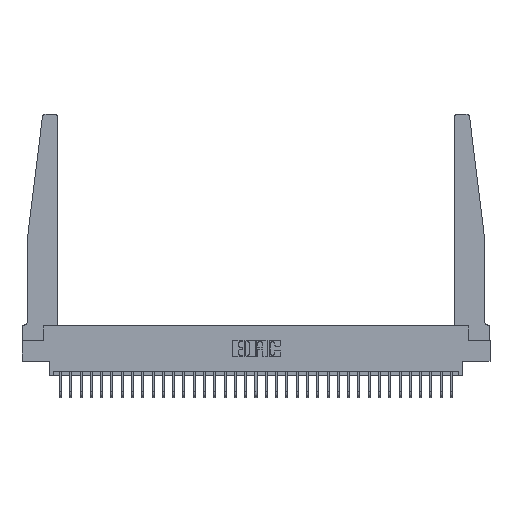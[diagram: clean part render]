
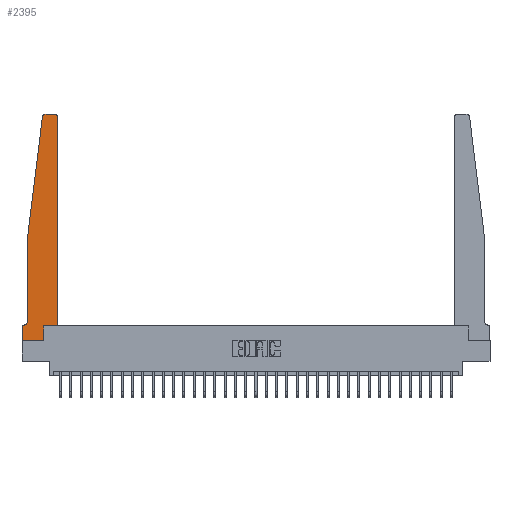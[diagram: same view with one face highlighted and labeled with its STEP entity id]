
A CAD part, top view. The second image highlights one B-rep face of the part: STEP entity #2395.
In plain terms, the highlighted planar face has unit normal (0, 0, 1).
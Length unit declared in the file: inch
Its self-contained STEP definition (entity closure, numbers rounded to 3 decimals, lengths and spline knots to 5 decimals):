
#1 = EDGE_CURVE ( 'NONE', #13689, #23639, #2510, .T. ) ;
#8 = DIRECTION ( 'NONE',  ( 0., 0., 1. ) ) ;
#1365 = ORIENTED_EDGE ( 'NONE', *, *, #23970, .T. ) ;
#1791 = EDGE_LOOP ( 'NONE', ( #9352, #6189, #14018, #2308, #9641, #16532, #23298, #17718, #9999, #11771, #1365, #20851 ) ) ;
#2158 = VERTEX_POINT ( 'NONE', #26513 ) ;
#2192 = DIRECTION ( 'NONE',  ( 0., 1., 0. ) ) ;
#2308 = ORIENTED_EDGE ( 'NONE', *, *, #10575, .T. ) ;
#2395 = ADVANCED_FACE ( 'NONE', ( #23514 ), #27385, .T. ) ;
#2459 = DIRECTION ( 'NONE',  ( -1., 0., 0. ) ) ;
#2510 = LINE ( 'NONE', #25712, #26073 ) ;
#2890 = AXIS2_PLACEMENT_3D ( 'NONE', #27079, #13449, #29350 ) ;
#3058 = VECTOR ( 'NONE', #11394, 39.37008 ) ;
#3444 = CARTESIAN_POINT ( 'NONE',  ( 0.015, 0.2375, 0.37 ) ) ;
#4073 = CARTESIAN_POINT ( 'NONE',  ( 0., 0., 0.37 ) ) ;
#4116 = EDGE_CURVE ( 'NONE', #18996, #13689, #15568, .T. ) ;
#4130 = AXIS2_PLACEMENT_3D ( 'NONE', #3444, #19445, #5785 ) ;
#5109 = VECTOR ( 'NONE', #2192, 39.37008 ) ;
#5785 = DIRECTION ( 'NONE',  ( -1., 0., 0. ) ) ;
#6189 = ORIENTED_EDGE ( 'NONE', *, *, #13111, .T. ) ;
#6371 = LINE ( 'NONE', #24095, #13177 ) ;
#6589 = EDGE_CURVE ( 'NONE', #14719, #13259, #29005, .T. ) ;
#7492 = CARTESIAN_POINT ( 'NONE',  ( 0.065, 1.25, 0.37 ) ) ;
#8091 = CARTESIAN_POINT ( 'NONE',  ( 0.395, 2.72, 0.37 ) ) ;
#8122 = DIRECTION ( 'NONE',  ( 0., -1., 0. ) ) ;
#8791 = VECTOR ( 'NONE', #26697, 39.37008 ) ;
#9352 = ORIENTED_EDGE ( 'NONE', *, *, #25266, .T. ) ;
#9641 = ORIENTED_EDGE ( 'NONE', *, *, #17659, .T. ) ;
#9794 = EDGE_CURVE ( 'NONE', #13259, #18996, #6371, .T. ) ;
#9999 = ORIENTED_EDGE ( 'NONE', *, *, #1, .T. ) ;
#10237 = DIRECTION ( 'NONE',  ( 1., 0., 0. ) ) ;
#10416 = DIRECTION ( 'NONE',  ( 1., 0., 0. ) ) ;
#10575 = EDGE_CURVE ( 'NONE', #20469, #19126, #15935, .T. ) ;
#11394 = DIRECTION ( 'NONE',  ( 0., -1., 0. ) ) ;
#11771 = ORIENTED_EDGE ( 'NONE', *, *, #29094, .T. ) ;
#11962 = EDGE_CURVE ( 'NONE', #21067, #12839, #21216, .T. ) ;
#12839 = VERTEX_POINT ( 'NONE', #27115 ) ;
#13071 = CARTESIAN_POINT ( 'NONE',  ( 0., 0., 0.37 ) ) ;
#13111 = EDGE_CURVE ( 'NONE', #2158, #23905, #21515, .T. ) ;
#13177 = VECTOR ( 'NONE', #8122, 39.37008 ) ;
#13259 = VERTEX_POINT ( 'NONE', #13929 ) ;
#13449 = DIRECTION ( 'NONE',  ( 0., 0., 1. ) ) ;
#13612 = CARTESIAN_POINT ( 'NONE',  ( 0.425, 0.18, 0.37 ) ) ;
#13689 = VERTEX_POINT ( 'NONE', #17655 ) ;
#13705 = CARTESIAN_POINT ( 'NONE',  ( 0.065, 0.2375, 0.37 ) ) ;
#13807 = VERTEX_POINT ( 'NONE', #13612 ) ;
#13882 = CARTESIAN_POINT ( 'NONE',  ( 0.25, 2.75, 0.37 ) ) ;
#13929 = CARTESIAN_POINT ( 'NONE',  ( 0., 0.1875, 0.37 ) ) ;
#14018 = ORIENTED_EDGE ( 'NONE', *, *, #21920, .T. ) ;
#14026 = CARTESIAN_POINT ( 'NONE',  ( 0.065, 0.1875, 0.37 ) ) ;
#14719 = VERTEX_POINT ( 'NONE', #16956 ) ;
#14818 = CARTESIAN_POINT ( 'NONE',  ( 0.2605, 0.18, 0.37 ) ) ;
#15162 = AXIS2_PLACEMENT_3D ( 'NONE', #27298, #8, #16016 ) ;
#15293 = CARTESIAN_POINT ( 'NONE',  ( 0.065, 1.25, 0.37 ) ) ;
#15568 = LINE ( 'NONE', #13071, #8791 ) ;
#15935 = LINE ( 'NONE', #15952, #3058 ) ;
#15952 = CARTESIAN_POINT ( 'NONE',  ( 0.065, 1.25, 0.37 ) ) ;
#16016 = DIRECTION ( 'NONE',  ( 1., 0., 0. ) ) ;
#16532 = ORIENTED_EDGE ( 'NONE', *, *, #6589, .T. ) ;
#16956 = CARTESIAN_POINT ( 'NONE',  ( 0.015, 0.1875, 0.37 ) ) ;
#16971 = VECTOR ( 'NONE', #17570, 39.37008 ) ;
#17080 = CARTESIAN_POINT ( 'NONE',  ( 0.425, 0.18, 0.37 ) ) ;
#17570 = DIRECTION ( 'NONE',  ( -0.122, -0.992, 0. ) ) ;
#17655 = CARTESIAN_POINT ( 'NONE',  ( 0.2605, 0., 0.37 ) ) ;
#17659 = EDGE_CURVE ( 'NONE', #19126, #14719, #19624, .T. ) ;
#17718 = ORIENTED_EDGE ( 'NONE', *, *, #4116, .T. ) ;
#17721 = LINE ( 'NONE', #15293, #16971 ) ;
#18054 = LINE ( 'NONE', #17080, #24840 ) ;
#18996 = VERTEX_POINT ( 'NONE', #4073 ) ;
#19126 = VERTEX_POINT ( 'NONE', #13705 ) ;
#19445 = DIRECTION ( 'NONE',  ( 0., 0., -1. ) ) ;
#19624 = CIRCLE ( 'NONE', #4130, 0.05 ) ;
#20469 = VERTEX_POINT ( 'NONE', #7492 ) ;
#20851 = ORIENTED_EDGE ( 'NONE', *, *, #11962, .T. ) ;
#20889 = DIRECTION ( 'NONE',  ( -1., 0., 0. ) ) ;
#21067 = VERTEX_POINT ( 'NONE', #26193 ) ;
#21216 = CIRCLE ( 'NONE', #25071, 0.03 ) ;
#21515 = CIRCLE ( 'NONE', #2890, 0.03 ) ;
#21920 = EDGE_CURVE ( 'NONE', #23905, #20469, #17721, .T. ) ;
#22965 = VECTOR ( 'NONE', #20889, 39.37008 ) ;
#23298 = ORIENTED_EDGE ( 'NONE', *, *, #9794, .T. ) ;
#23514 = FACE_OUTER_BOUND ( 'NONE', #1791, .T. ) ;
#23572 = LINE ( 'NONE', #13882, #28904 ) ;
#23639 = VERTEX_POINT ( 'NONE', #14818 ) ;
#23905 = VERTEX_POINT ( 'NONE', #24660 ) ;
#23970 = EDGE_CURVE ( 'NONE', #13807, #21067, #28647, .T. ) ;
#24069 = DIRECTION ( 'NONE',  ( 0., 0., 1. ) ) ;
#24095 = CARTESIAN_POINT ( 'NONE',  ( 0., 0., 0.37 ) ) ;
#24660 = CARTESIAN_POINT ( 'NONE',  ( 0.24675, 2.72367, 0.37 ) ) ;
#24840 = VECTOR ( 'NONE', #10237, 39.37008 ) ;
#24952 = CARTESIAN_POINT ( 'NONE',  ( 0.425, 0.18, 0.37 ) ) ;
#25071 = AXIS2_PLACEMENT_3D ( 'NONE', #8091, #24069, #10416 ) ;
#25266 = EDGE_CURVE ( 'NONE', #12839, #2158, #23572, .T. ) ;
#25712 = CARTESIAN_POINT ( 'NONE',  ( 0.2605, 0.18, 0.37 ) ) ;
#26073 = VECTOR ( 'NONE', #27790, 39.37008 ) ;
#26193 = CARTESIAN_POINT ( 'NONE',  ( 0.425, 2.72, 0.37 ) ) ;
#26513 = CARTESIAN_POINT ( 'NONE',  ( 0.27653, 2.75, 0.37 ) ) ;
#26697 = DIRECTION ( 'NONE',  ( 1., 0., 0. ) ) ;
#27079 = CARTESIAN_POINT ( 'NONE',  ( 0.27653, 2.72, 0.37 ) ) ;
#27115 = CARTESIAN_POINT ( 'NONE',  ( 0.395, 2.75, 0.37 ) ) ;
#27298 = CARTESIAN_POINT ( 'NONE',  ( 0., 0.1875, 0.37 ) ) ;
#27385 = PLANE ( 'NONE',  #15162 ) ;
#27790 = DIRECTION ( 'NONE',  ( 0., 1., 0. ) ) ;
#28647 = LINE ( 'NONE', #24952, #5109 ) ;
#28904 = VECTOR ( 'NONE', #2459, 39.37008 ) ;
#29005 = LINE ( 'NONE', #14026, #22965 ) ;
#29094 = EDGE_CURVE ( 'NONE', #23639, #13807, #18054, .T. ) ;
#29350 = DIRECTION ( 'NONE',  ( 1., 0., 0. ) ) ;
